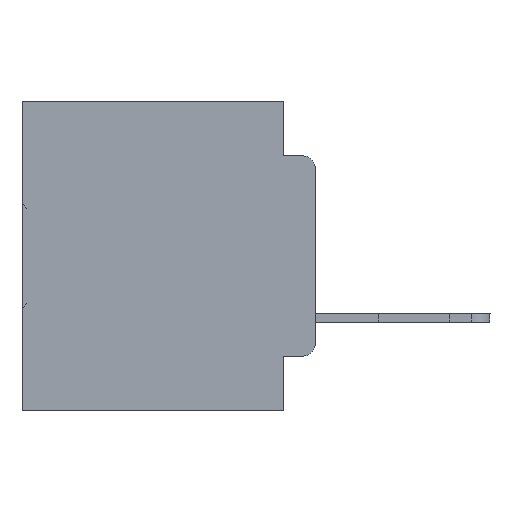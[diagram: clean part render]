
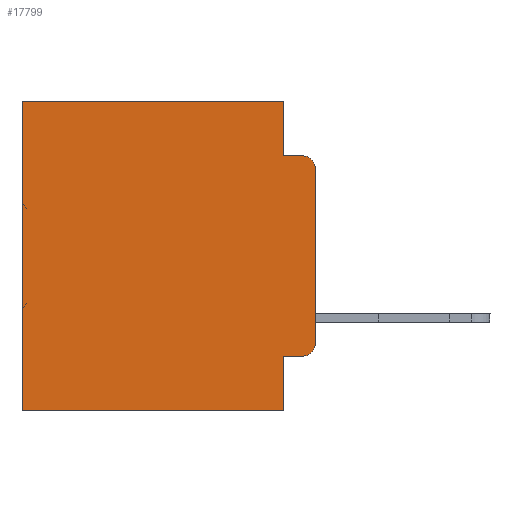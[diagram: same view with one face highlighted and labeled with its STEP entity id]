
A CAD part, left-side view. The second image highlights one B-rep face of the part: STEP entity #17799.
In plain terms, the highlighted planar face has unit normal (-1, 0, 0).
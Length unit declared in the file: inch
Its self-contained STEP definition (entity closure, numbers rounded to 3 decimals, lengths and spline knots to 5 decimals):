
#55 = CARTESIAN_POINT ( 'NONE',  ( 0.298, 0.051, -0.4115 ) ) ;
#164 = ORIENTED_EDGE ( 'NONE', *, *, #6066, .T. ) ;
#349 = ORIENTED_EDGE ( 'NONE', *, *, #5724, .T. ) ;
#1308 = DIRECTION ( 'NONE',  ( 0., -1., 0. ) ) ;
#1530 = VECTOR ( 'NONE', #31076, 39.37008 ) ;
#2467 = DIRECTION ( 'NONE',  ( 0., 1., 0. ) ) ;
#2567 = ORIENTED_EDGE ( 'NONE', *, *, #20888, .F. ) ;
#2590 = CARTESIAN_POINT ( 'NONE',  ( 0.298, 0., 0. ) ) ;
#2664 = VERTEX_POINT ( 'NONE', #31403 ) ;
#3254 = VERTEX_POINT ( 'NONE', #30168 ) ;
#4061 = LINE ( 'NONE', #20377, #29401 ) ;
#4062 = CARTESIAN_POINT ( 'NONE',  ( 0.298, 0.051, -0.0885 ) ) ;
#4143 = PLANE ( 'NONE',  #4907 ) ;
#4160 = CARTESIAN_POINT ( 'NONE',  ( 0.298, 0.051, -0.4115 ) ) ;
#4173 = DIRECTION ( 'NONE',  ( 0., 0., -1. ) ) ;
#4626 = DIRECTION ( 'NONE',  ( -1., 0., 0. ) ) ;
#4907 = AXIS2_PLACEMENT_3D ( 'NONE', #25634, #22803, #22683 ) ;
#5039 = CIRCLE ( 'NONE', #8198, 0.02 ) ;
#5081 = DIRECTION ( 'NONE',  ( 0., 0., -1. ) ) ;
#5724 = EDGE_CURVE ( 'NONE', #9673, #11133, #33573, .T. ) ;
#5925 = ORIENTED_EDGE ( 'NONE', *, *, #29721, .T. ) ;
#6066 = EDGE_CURVE ( 'NONE', #11133, #6720, #8705, .T. ) ;
#6720 = VERTEX_POINT ( 'NONE', #30171 ) ;
#6817 = EDGE_CURVE ( 'NONE', #10805, #2664, #25117, .T. ) ;
#7166 = ORIENTED_EDGE ( 'NONE', *, *, #7670, .F. ) ;
#7388 = VECTOR ( 'NONE', #2467, 39.37008 ) ;
#7665 = CARTESIAN_POINT ( 'NONE',  ( 0.298, 0., 0. ) ) ;
#7670 = EDGE_CURVE ( 'NONE', #17832, #6720, #34348, .T. ) ;
#8198 = AXIS2_PLACEMENT_3D ( 'NONE', #21169, #4626, #12502 ) ;
#8530 = VERTEX_POINT ( 'NONE', #55 ) ;
#8561 = LINE ( 'NONE', #4062, #28414 ) ;
#8657 = VERTEX_POINT ( 'NONE', #27547 ) ;
#8705 = LINE ( 'NONE', #20534, #1530 ) ;
#9673 = VERTEX_POINT ( 'NONE', #24962 ) ;
#10028 = DIRECTION ( 'NONE',  ( 0., 0., -1. ) ) ;
#10805 = VERTEX_POINT ( 'NONE', #30777 ) ;
#11133 = VERTEX_POINT ( 'NONE', #33339 ) ;
#11737 = EDGE_CURVE ( 'NONE', #16762, #2664, #15513, .T. ) ;
#12320 = EDGE_CURVE ( 'NONE', #9673, #8657, #4061, .T. ) ;
#12502 = DIRECTION ( 'NONE',  ( 0., 0., -1. ) ) ;
#12974 = VECTOR ( 'NONE', #33868, 39.37008 ) ;
#13443 = DIRECTION ( 'NONE',  ( 0., 1., 0. ) ) ;
#15505 = CARTESIAN_POINT ( 'NONE',  ( 0.298, 0.051, -0.5 ) ) ;
#15513 = CIRCLE ( 'NONE', #16047, 0.02 ) ;
#15527 = LINE ( 'NONE', #23218, #12974 ) ;
#16047 = AXIS2_PLACEMENT_3D ( 'NONE', #26176, #31077, #10028 ) ;
#16762 = VERTEX_POINT ( 'NONE', #17317 ) ;
#17299 = ORIENTED_EDGE ( 'NONE', *, *, #6817, .F. ) ;
#17317 = CARTESIAN_POINT ( 'NONE',  ( 0.298, 0.02, -0.4115 ) ) ;
#17799 = ADVANCED_FACE ( 'NONE', ( #32545 ), #4143, .F. ) ;
#17832 = VERTEX_POINT ( 'NONE', #15505 ) ;
#20266 = EDGE_CURVE ( 'NONE', #10805, #3254, #5039, .T. ) ;
#20377 = CARTESIAN_POINT ( 'NONE',  ( 0.298, 0.051, 0. ) ) ;
#20534 = CARTESIAN_POINT ( 'NONE',  ( 0.298, 0.473, 0. ) ) ;
#20888 = EDGE_CURVE ( 'NONE', #8530, #17832, #15527, .T. ) ;
#21169 = CARTESIAN_POINT ( 'NONE',  ( 0.298, 0.02, -0.1085 ) ) ;
#22683 = DIRECTION ( 'NONE',  ( 0., 0., -1. ) ) ;
#22803 = DIRECTION ( 'NONE',  ( 1., 0., 0. ) ) ;
#23084 = DIRECTION ( 'NONE',  ( 0., -1., 0. ) ) ;
#23218 = CARTESIAN_POINT ( 'NONE',  ( 0.298, 0.051, 0. ) ) ;
#23254 = VECTOR ( 'NONE', #23084, 39.37008 ) ;
#24008 = CARTESIAN_POINT ( 'NONE',  ( 0.298, 0., -0.5 ) ) ;
#24755 = ORIENTED_EDGE ( 'NONE', *, *, #11737, .T. ) ;
#24962 = CARTESIAN_POINT ( 'NONE',  ( 0.298, 0.051, 0. ) ) ;
#25117 = LINE ( 'NONE', #7665, #28507 ) ;
#25634 = CARTESIAN_POINT ( 'NONE',  ( 0.298, 0., 0. ) ) ;
#25864 = ORIENTED_EDGE ( 'NONE', *, *, #12320, .F. ) ;
#26176 = CARTESIAN_POINT ( 'NONE',  ( 0.298, 0.02, -0.3915 ) ) ;
#26221 = EDGE_LOOP ( 'NONE', ( #17299, #26948, #28676, #25864, #349, #164, #7166, #2567, #5925, #24755 ) ) ;
#26477 = VECTOR ( 'NONE', #13443, 39.37008 ) ;
#26948 = ORIENTED_EDGE ( 'NONE', *, *, #20266, .T. ) ;
#27203 = EDGE_CURVE ( 'NONE', #8657, #3254, #8561, .T. ) ;
#27547 = CARTESIAN_POINT ( 'NONE',  ( 0.298, 0.051, -0.0885 ) ) ;
#28414 = VECTOR ( 'NONE', #1308, 39.37008 ) ;
#28507 = VECTOR ( 'NONE', #5081, 39.37008 ) ;
#28676 = ORIENTED_EDGE ( 'NONE', *, *, #27203, .F. ) ;
#29401 = VECTOR ( 'NONE', #4173, 39.37008 ) ;
#29721 = EDGE_CURVE ( 'NONE', #8530, #16762, #33725, .T. ) ;
#30168 = CARTESIAN_POINT ( 'NONE',  ( 0.298, 0.02, -0.0885 ) ) ;
#30171 = CARTESIAN_POINT ( 'NONE',  ( 0.298, 0.473, -0.5 ) ) ;
#30777 = CARTESIAN_POINT ( 'NONE',  ( 0.298, 0., -0.1085 ) ) ;
#31076 = DIRECTION ( 'NONE',  ( 0., 0., -1. ) ) ;
#31077 = DIRECTION ( 'NONE',  ( -1., 0., 0. ) ) ;
#31403 = CARTESIAN_POINT ( 'NONE',  ( 0.298, 0., -0.3915 ) ) ;
#32545 = FACE_OUTER_BOUND ( 'NONE', #26221, .T. ) ;
#33339 = CARTESIAN_POINT ( 'NONE',  ( 0.298, 0.473, 0. ) ) ;
#33573 = LINE ( 'NONE', #2590, #26477 ) ;
#33725 = LINE ( 'NONE', #4160, #23254 ) ;
#33868 = DIRECTION ( 'NONE',  ( 0., 0., -1. ) ) ;
#34348 = LINE ( 'NONE', #24008, #7388 ) ;
